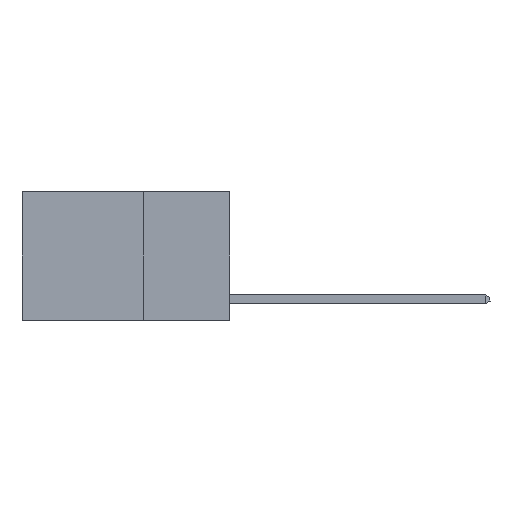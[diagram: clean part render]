
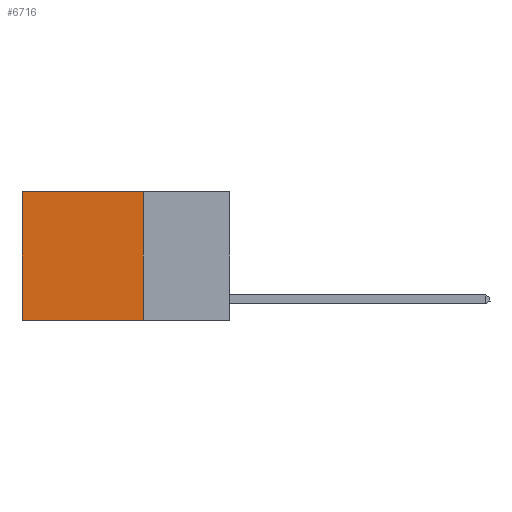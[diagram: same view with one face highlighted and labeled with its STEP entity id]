
A CAD part, left-side view. The second image highlights one B-rep face of the part: STEP entity #6716.
In plain terms, the highlighted planar face has unit normal (-1, 0, 0).
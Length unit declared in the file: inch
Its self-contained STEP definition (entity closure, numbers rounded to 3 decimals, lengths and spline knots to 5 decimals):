
#560 = VERTEX_POINT ( 'NONE', #18918 ) ;
#949 = CARTESIAN_POINT ( 'NONE',  ( 0.2625, 0.25, -0.37 ) ) ;
#1719 = DIRECTION ( 'NONE',  ( 0., 0., -1. ) ) ;
#1800 = CARTESIAN_POINT ( 'NONE',  ( 0.2625, 0.6, 0. ) ) ;
#2285 = VECTOR ( 'NONE', #7148, 39.37008 ) ;
#3634 = LINE ( 'NONE', #5495, #2285 ) ;
#4405 = VECTOR ( 'NONE', #5342, 39.37008 ) ;
#5342 = DIRECTION ( 'NONE',  ( 0., 1., 0. ) ) ;
#5495 = CARTESIAN_POINT ( 'NONE',  ( 0.2625, 0.25, 0. ) ) ;
#5497 = AXIS2_PLACEMENT_3D ( 'NONE', #10000, #14970, #1719 ) ;
#6082 = EDGE_LOOP ( 'NONE', ( #16254, #13718, #10228, #21072 ) ) ;
#6716 = ADVANCED_FACE ( 'NONE', ( #11641 ), #18149, .F. ) ;
#7051 = VERTEX_POINT ( 'NONE', #19637 ) ;
#7148 = DIRECTION ( 'NONE',  ( 0., 0., -1. ) ) ;
#7178 = EDGE_CURVE ( 'NONE', #7051, #8264, #15065, .T. ) ;
#7330 = VERTEX_POINT ( 'NONE', #20302 ) ;
#8264 = VERTEX_POINT ( 'NONE', #10274 ) ;
#8823 = CARTESIAN_POINT ( 'NONE',  ( 0.2625, 0.25, 0. ) ) ;
#10000 = CARTESIAN_POINT ( 'NONE',  ( 0.2625, 0.25, 0. ) ) ;
#10196 = DIRECTION ( 'NONE',  ( 0., 0., -1. ) ) ;
#10228 = ORIENTED_EDGE ( 'NONE', *, *, #11477, .F. ) ;
#10274 = CARTESIAN_POINT ( 'NONE',  ( 0.2625, 0.6, -0.37 ) ) ;
#11477 = EDGE_CURVE ( 'NONE', #7330, #560, #3634, .T. ) ;
#11641 = FACE_OUTER_BOUND ( 'NONE', #6082, .T. ) ;
#13661 = LINE ( 'NONE', #8823, #4405 ) ;
#13718 = ORIENTED_EDGE ( 'NONE', *, *, #18359, .F. ) ;
#13938 = VECTOR ( 'NONE', #21005, 39.37008 ) ;
#14970 = DIRECTION ( 'NONE',  ( 1., 0., 0. ) ) ;
#15065 = LINE ( 'NONE', #1800, #18110 ) ;
#15950 = LINE ( 'NONE', #949, #13938 ) ;
#16254 = ORIENTED_EDGE ( 'NONE', *, *, #7178, .T. ) ;
#18110 = VECTOR ( 'NONE', #10196, 39.37008 ) ;
#18149 = PLANE ( 'NONE',  #5497 ) ;
#18359 = EDGE_CURVE ( 'NONE', #560, #8264, #15950, .T. ) ;
#18918 = CARTESIAN_POINT ( 'NONE',  ( 0.2625, 0.25, -0.37 ) ) ;
#19637 = CARTESIAN_POINT ( 'NONE',  ( 0.2625, 0.6, 0. ) ) ;
#20302 = CARTESIAN_POINT ( 'NONE',  ( 0.2625, 0.25, 0. ) ) ;
#21005 = DIRECTION ( 'NONE',  ( 0., 1., 0. ) ) ;
#21072 = ORIENTED_EDGE ( 'NONE', *, *, #21349, .T. ) ;
#21349 = EDGE_CURVE ( 'NONE', #7330, #7051, #13661, .T. ) ;
